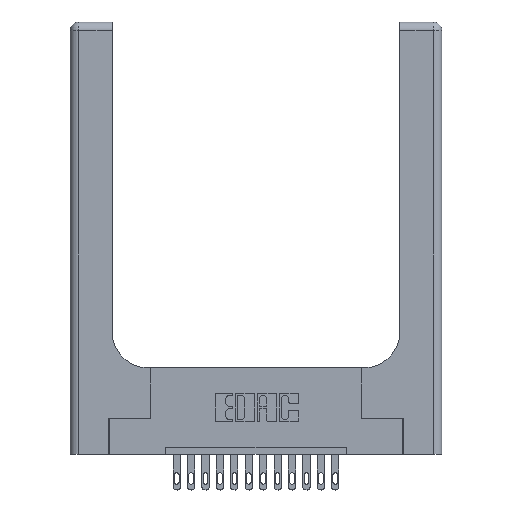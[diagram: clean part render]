
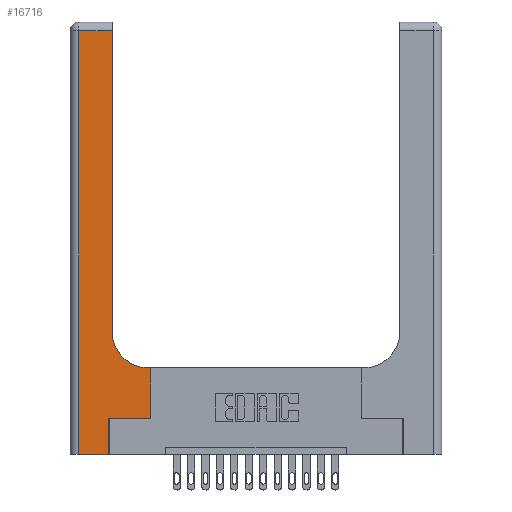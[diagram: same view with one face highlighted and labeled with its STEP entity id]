
A CAD part, top view. The second image highlights one B-rep face of the part: STEP entity #16716.
In plain terms, the highlighted planar face has unit normal (0, 0, 1).
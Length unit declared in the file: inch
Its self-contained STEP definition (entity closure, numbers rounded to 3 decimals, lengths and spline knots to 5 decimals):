
#12 = CARTESIAN_POINT ( 'NONE',  ( 0.5585, 0.25, 0.37 ) ) ;
#37 = ORIENTED_EDGE ( 'NONE', *, *, #15090, .T. ) ;
#370 = VECTOR ( 'NONE', #9788, 39.37008 ) ;
#644 = EDGE_CURVE ( 'NONE', #11648, #11158, #11785, .T. ) ;
#1176 = DIRECTION ( 'NONE',  ( 1., 0., 0. ) ) ;
#1210 = VERTEX_POINT ( 'NONE', #5459 ) ;
#1344 = CARTESIAN_POINT ( 'NONE',  ( 0.5585, 0.6, 0.37 ) ) ;
#1563 = ORIENTED_EDGE ( 'NONE', *, *, #644, .T. ) ;
#1777 = CARTESIAN_POINT ( 'NONE',  ( 0., 2.94, 0.37 ) ) ;
#2012 = EDGE_CURVE ( 'NONE', #4645, #5656, #7274, .T. ) ;
#2488 = VECTOR ( 'NONE', #6937, 39.37008 ) ;
#2807 = VECTOR ( 'NONE', #10526, 39.37008 ) ;
#3329 = ORIENTED_EDGE ( 'NONE', *, *, #12283, .T. ) ;
#3541 = VECTOR ( 'NONE', #15882, 39.37008 ) ;
#3879 = EDGE_CURVE ( 'NONE', #9156, #15019, #15519, .T. ) ;
#3990 = LINE ( 'NONE', #1777, #3541 ) ;
#4117 = CARTESIAN_POINT ( 'NONE',  ( 0.5585, 0.25, 0.37 ) ) ;
#4133 = CARTESIAN_POINT ( 'NONE',  ( 0., 0., 0.37 ) ) ;
#4215 = EDGE_CURVE ( 'NONE', #5656, #11648, #11128, .T. ) ;
#4645 = VERTEX_POINT ( 'NONE', #15484 ) ;
#5174 = CIRCLE ( 'NONE', #6801, 0.25 ) ;
#5236 = CARTESIAN_POINT ( 'NONE',  ( 0.269, 0.25, 0.37 ) ) ;
#5335 = EDGE_CURVE ( 'NONE', #8398, #1210, #10232, .T. ) ;
#5459 = CARTESIAN_POINT ( 'NONE',  ( 0.5415, 0.6, 0.37 ) ) ;
#5656 = VERTEX_POINT ( 'NONE', #13278 ) ;
#6491 = CARTESIAN_POINT ( 'NONE',  ( 0.2915, 3., 0.37 ) ) ;
#6580 = DIRECTION ( 'NONE',  ( 0., 0., -1. ) ) ;
#6801 = AXIS2_PLACEMENT_3D ( 'NONE', #17798, #6580, #16377 ) ;
#6937 = DIRECTION ( 'NONE',  ( 0., 1., 0. ) ) ;
#7274 = LINE ( 'NONE', #4133, #12750 ) ;
#7300 = PLANE ( 'NONE',  #9990 ) ;
#7356 = ORIENTED_EDGE ( 'NONE', *, *, #5335, .T. ) ;
#7412 = VECTOR ( 'NONE', #1176, 39.37008 ) ;
#7786 = LINE ( 'NONE', #10000, #11285 ) ;
#8398 = VERTEX_POINT ( 'NONE', #1344 ) ;
#8646 = DIRECTION ( 'NONE',  ( 1., 0., 0. ) ) ;
#8700 = CARTESIAN_POINT ( 'NONE',  ( 0., 3., 0.37 ) ) ;
#9156 = VERTEX_POINT ( 'NONE', #17729 ) ;
#9788 = DIRECTION ( 'NONE',  ( 0., 1., 0. ) ) ;
#9870 = DIRECTION ( 'NONE',  ( 0., -1., 0. ) ) ;
#9990 = AXIS2_PLACEMENT_3D ( 'NONE', #8700, #10097, #11341 ) ;
#10000 = CARTESIAN_POINT ( 'NONE',  ( 0.06, 3., 0.37 ) ) ;
#10097 = DIRECTION ( 'NONE',  ( 0., 0., -1. ) ) ;
#10232 = LINE ( 'NONE', #12207, #13537 ) ;
#10525 = EDGE_LOOP ( 'NONE', ( #11209, #37, #15117, #17867, #16271, #1563, #3329, #7356, #15475 ) ) ;
#10526 = DIRECTION ( 'NONE',  ( 0., 1., 0. ) ) ;
#11057 = CARTESIAN_POINT ( 'NONE',  ( 0.269, 0.25, 0.37 ) ) ;
#11128 = LINE ( 'NONE', #16920, #370 ) ;
#11145 = VERTEX_POINT ( 'NONE', #16837 ) ;
#11158 = VERTEX_POINT ( 'NONE', #12 ) ;
#11209 = ORIENTED_EDGE ( 'NONE', *, *, #3879, .T. ) ;
#11285 = VECTOR ( 'NONE', #9870, 39.37008 ) ;
#11341 = DIRECTION ( 'NONE',  ( -1., 0., 0. ) ) ;
#11648 = VERTEX_POINT ( 'NONE', #5236 ) ;
#11663 = EDGE_CURVE ( 'NONE', #1210, #9156, #5174, .T. ) ;
#11785 = LINE ( 'NONE', #11057, #7412 ) ;
#12207 = CARTESIAN_POINT ( 'NONE',  ( 0.2915, 0.6, 0.37 ) ) ;
#12283 = EDGE_CURVE ( 'NONE', #11158, #8398, #15212, .T. ) ;
#12750 = VECTOR ( 'NONE', #8646, 39.37008 ) ;
#13278 = CARTESIAN_POINT ( 'NONE',  ( 0.269, 0., 0.37 ) ) ;
#13537 = VECTOR ( 'NONE', #13638, 39.37008 ) ;
#13638 = DIRECTION ( 'NONE',  ( -1., 0., 0. ) ) ;
#15019 = VERTEX_POINT ( 'NONE', #16898 ) ;
#15090 = EDGE_CURVE ( 'NONE', #15019, #11145, #3990, .T. ) ;
#15117 = ORIENTED_EDGE ( 'NONE', *, *, #15898, .T. ) ;
#15212 = LINE ( 'NONE', #4117, #2488 ) ;
#15475 = ORIENTED_EDGE ( 'NONE', *, *, #11663, .T. ) ;
#15484 = CARTESIAN_POINT ( 'NONE',  ( 0.06, 0., 0.37 ) ) ;
#15519 = LINE ( 'NONE', #6491, #2807 ) ;
#15882 = DIRECTION ( 'NONE',  ( -1., 0., 0. ) ) ;
#15898 = EDGE_CURVE ( 'NONE', #11145, #4645, #7786, .T. ) ;
#16271 = ORIENTED_EDGE ( 'NONE', *, *, #4215, .T. ) ;
#16377 = DIRECTION ( 'NONE',  ( 1., 0., 0. ) ) ;
#16716 = ADVANCED_FACE ( 'NONE', ( #17176 ), #7300, .F. ) ;
#16837 = CARTESIAN_POINT ( 'NONE',  ( 0.06, 2.94, 0.37 ) ) ;
#16898 = CARTESIAN_POINT ( 'NONE',  ( 0.2915, 2.94, 0.37 ) ) ;
#16920 = CARTESIAN_POINT ( 'NONE',  ( 0.269, 0., 0.37 ) ) ;
#17176 = FACE_OUTER_BOUND ( 'NONE', #10525, .T. ) ;
#17729 = CARTESIAN_POINT ( 'NONE',  ( 0.2915, 0.85, 0.37 ) ) ;
#17798 = CARTESIAN_POINT ( 'NONE',  ( 0.5415, 0.85, 0.37 ) ) ;
#17867 = ORIENTED_EDGE ( 'NONE', *, *, #2012, .T. ) ;
